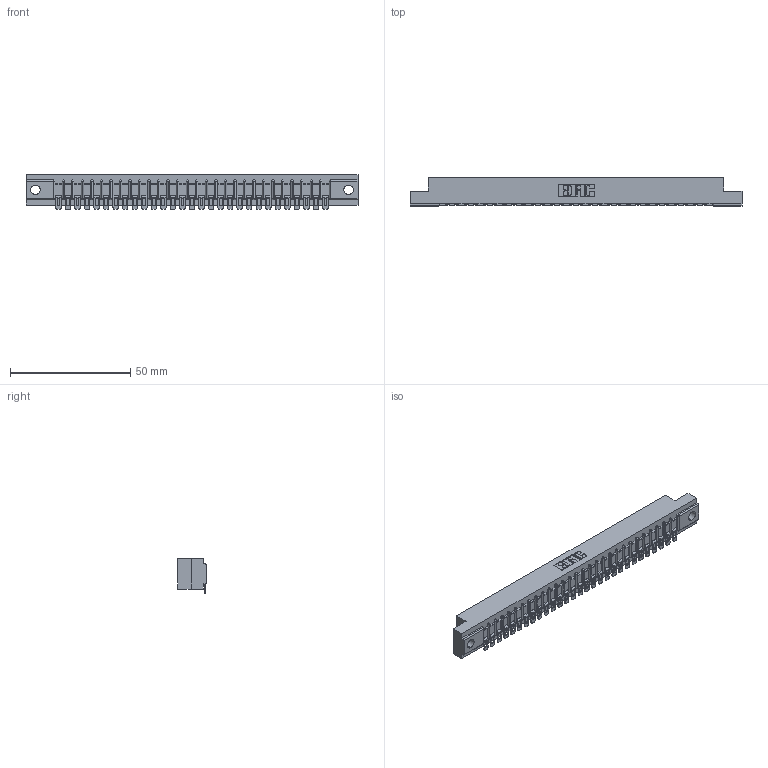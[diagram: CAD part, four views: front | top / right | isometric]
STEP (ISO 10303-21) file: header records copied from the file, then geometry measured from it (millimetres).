
FILE_DESCRIPTION (( 'STEP AP203' ), '1' );
FILE_NAME ('357-029-454-104.STEP', '2020-10-01T23:58:53', ( '' ), ( '' ), 'SwSTEP 2.0', 'SolidWorks 2020', '' );
FILE_SCHEMA (( 'CONFIG_CONTROL_DESIGN' ));
Length unit declared in the file: inch
Products named in the file (3): 307-290-002_554; 307 Part_.156 Dia Mounting Holes; 357-029-454-104
Assembly tree (30 placements, depth 2):
  357-029-454-104
    307 Part_.156 Dia Mounting Holes
    307-290-002_554  x29
Bounding box: 137.92 x 12.01 x 14.52 mm (x, y, z)
Volume: 14567 mm3; surface area: 17978.9 mm2
Topology: 30 solids, 30 shells, 2511 faces, 7696 edges, 5048 vertices
Faces by surface type: plane 1418, cylinder 1033, sphere 60
Entity records: 27847 total; most frequent: CARTESIAN_POINT 4700, ORIENTED_EDGE 4688, DIRECTION 4570, EDGE_CURVE 2344, VECTOR 1790, LINE 1790, VERTEX_POINT 1520, AXIS2_PLACEMENT_3D 1390
